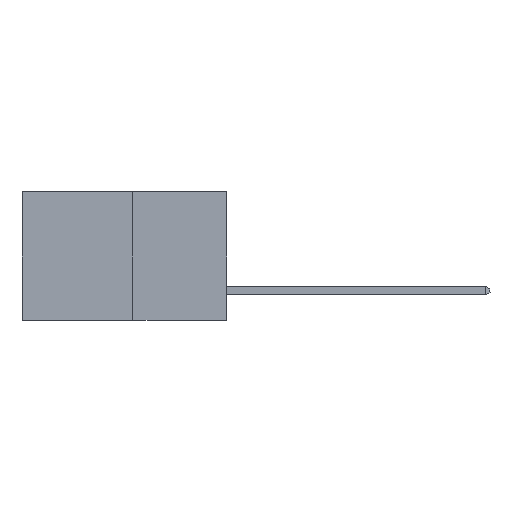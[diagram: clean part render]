
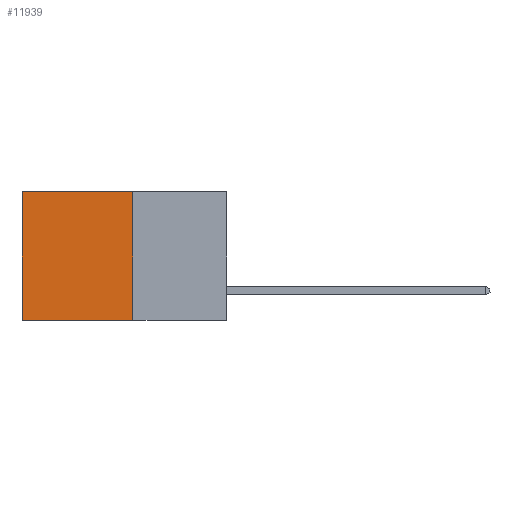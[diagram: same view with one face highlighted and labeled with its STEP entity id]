
A CAD part, left-side view. The second image highlights one B-rep face of the part: STEP entity #11939.
In plain terms, the highlighted planar face has unit normal (-1, 0, 0).
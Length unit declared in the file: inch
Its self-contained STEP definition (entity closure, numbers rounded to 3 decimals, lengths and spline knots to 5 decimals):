
#200 = VERTEX_POINT ( 'NONE', #10154 ) ;
#401 = LINE ( 'NONE', #7602, #6302 ) ;
#1173 = DIRECTION ( 'NONE',  ( 0., 0., -1. ) ) ;
#1384 = CARTESIAN_POINT ( 'NONE',  ( 0.277, 0.27, 0. ) ) ;
#1399 = PLANE ( 'NONE',  #9247 ) ;
#1615 = EDGE_CURVE ( 'NONE', #8413, #200, #401, .T. ) ;
#2685 = LINE ( 'NONE', #6297, #11323 ) ;
#3142 = CARTESIAN_POINT ( 'NONE',  ( 0.277, 0.59, 0. ) ) ;
#3561 = EDGE_LOOP ( 'NONE', ( #4795, #7320, #4614, #12142 ) ) ;
#4068 = CARTESIAN_POINT ( 'NONE',  ( 0.277, 0.27, 0. ) ) ;
#4614 = ORIENTED_EDGE ( 'NONE', *, *, #7433, .F. ) ;
#4795 = ORIENTED_EDGE ( 'NONE', *, *, #1615, .T. ) ;
#4796 = EDGE_CURVE ( 'NONE', #11067, #200, #2685, .T. ) ;
#4926 = CARTESIAN_POINT ( 'NONE',  ( 0.277, 0.27, -0.37 ) ) ;
#5463 = EDGE_CURVE ( 'NONE', #10623, #8413, #6270, .T. ) ;
#6022 = LINE ( 'NONE', #9233, #8690 ) ;
#6087 = DIRECTION ( 'NONE',  ( 1., 0., 0. ) ) ;
#6270 = LINE ( 'NONE', #4068, #6611 ) ;
#6297 = CARTESIAN_POINT ( 'NONE',  ( 0.277, 0.27, -0.37 ) ) ;
#6302 = VECTOR ( 'NONE', #7620, 39.37008 ) ;
#6611 = VECTOR ( 'NONE', #11881, 39.37008 ) ;
#7037 = FACE_OUTER_BOUND ( 'NONE', #3561, .T. ) ;
#7320 = ORIENTED_EDGE ( 'NONE', *, *, #4796, .F. ) ;
#7433 = EDGE_CURVE ( 'NONE', #10623, #11067, #6022, .T. ) ;
#7450 = DIRECTION ( 'NONE',  ( 0., 1., 0. ) ) ;
#7602 = CARTESIAN_POINT ( 'NONE',  ( 0.277, 0.59, -0.37 ) ) ;
#7620 = DIRECTION ( 'NONE',  ( 0., 0., -1. ) ) ;
#8413 = VERTEX_POINT ( 'NONE', #3142 ) ;
#8690 = VECTOR ( 'NONE', #1173, 39.37008 ) ;
#9233 = CARTESIAN_POINT ( 'NONE',  ( 0.277, 0.27, -0.37 ) ) ;
#9247 = AXIS2_PLACEMENT_3D ( 'NONE', #4926, #6087, #13794 ) ;
#10154 = CARTESIAN_POINT ( 'NONE',  ( 0.277, 0.59, -0.37 ) ) ;
#10623 = VERTEX_POINT ( 'NONE', #1384 ) ;
#11067 = VERTEX_POINT ( 'NONE', #14432 ) ;
#11323 = VECTOR ( 'NONE', #7450, 39.37008 ) ;
#11881 = DIRECTION ( 'NONE',  ( 0., 1., 0. ) ) ;
#11939 = ADVANCED_FACE ( 'NONE', ( #7037 ), #1399, .F. ) ;
#12142 = ORIENTED_EDGE ( 'NONE', *, *, #5463, .T. ) ;
#13794 = DIRECTION ( 'NONE',  ( 0., 0., -1. ) ) ;
#14432 = CARTESIAN_POINT ( 'NONE',  ( 0.277, 0.27, -0.37 ) ) ;
